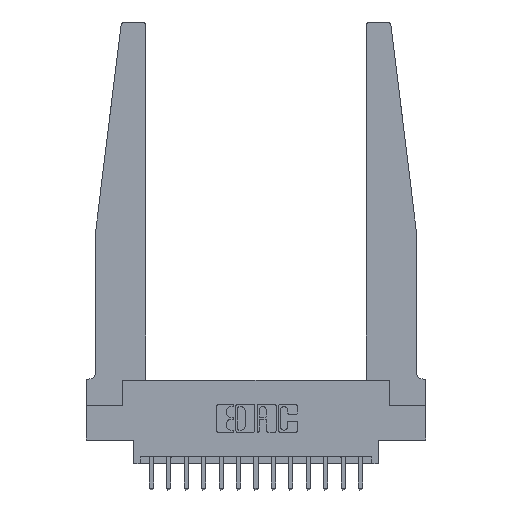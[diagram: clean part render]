
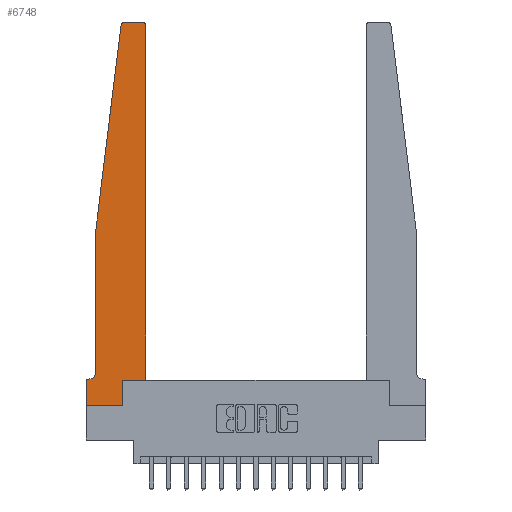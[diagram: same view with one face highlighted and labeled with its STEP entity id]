
A CAD part, top view. The second image highlights one B-rep face of the part: STEP entity #6748.
In plain terms, the highlighted planar face has unit normal (0, 0, 1).
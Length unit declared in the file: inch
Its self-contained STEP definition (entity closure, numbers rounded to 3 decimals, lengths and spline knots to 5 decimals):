
#84 = VERTEX_POINT ( 'NONE', #8165 ) ;
#368 = ORIENTED_EDGE ( 'NONE', *, *, #16164, .T. ) ;
#447 = VERTEX_POINT ( 'NONE', #3151 ) ;
#698 = CARTESIAN_POINT ( 'NONE',  ( 0.065, 0.1875, 0.37 ) ) ;
#712 = CARTESIAN_POINT ( 'NONE',  ( 0.27653, 2.75, 0.37 ) ) ;
#878 = EDGE_CURVE ( 'NONE', #8238, #4506, #9283, .T. ) ;
#1342 = DIRECTION ( 'NONE',  ( 1., 0., 0. ) ) ;
#1402 = AXIS2_PLACEMENT_3D ( 'NONE', #2797, #12107, #4126 ) ;
#1645 = ORIENTED_EDGE ( 'NONE', *, *, #16188, .T. ) ;
#1782 = CARTESIAN_POINT ( 'NONE',  ( 0.25, 2.75, 0.37 ) ) ;
#2006 = EDGE_CURVE ( 'NONE', #3058, #6667, #7144, .T. ) ;
#2750 = CARTESIAN_POINT ( 'NONE',  ( 0.425, 0.18, 0.37 ) ) ;
#2772 = CARTESIAN_POINT ( 'NONE',  ( 0., 0., 0.37 ) ) ;
#2797 = CARTESIAN_POINT ( 'NONE',  ( 0., 0.1875, 0.37 ) ) ;
#3058 = VERTEX_POINT ( 'NONE', #8673 ) ;
#3151 = CARTESIAN_POINT ( 'NONE',  ( 0.015, 0.1875, 0.37 ) ) ;
#3256 = DIRECTION ( 'NONE',  ( 1., 0., 0. ) ) ;
#4053 = EDGE_CURVE ( 'NONE', #12552, #5627, #13648, .T. ) ;
#4085 = DIRECTION ( 'NONE',  ( 0., 1., 0. ) ) ;
#4126 = DIRECTION ( 'NONE',  ( 1., 0., 0. ) ) ;
#4337 = ORIENTED_EDGE ( 'NONE', *, *, #11770, .T. ) ;
#4506 = VERTEX_POINT ( 'NONE', #17321 ) ;
#4568 = AXIS2_PLACEMENT_3D ( 'NONE', #10434, #10341, #10271 ) ;
#4741 = CIRCLE ( 'NONE', #15214, 0.05 ) ;
#4788 = EDGE_LOOP ( 'NONE', ( #9194, #16767, #4337, #1645, #368, #7497, #8402, #14737, #12837, #5644, #10534, #6061 ) ) ;
#4977 = DIRECTION ( 'NONE',  ( 0., 0., -1. ) ) ;
#5025 = CARTESIAN_POINT ( 'NONE',  ( 0., 0.1875, 0.37 ) ) ;
#5384 = CARTESIAN_POINT ( 'NONE',  ( 0.065, 1.25, 0.37 ) ) ;
#5473 = VERTEX_POINT ( 'NONE', #5384 ) ;
#5627 = VERTEX_POINT ( 'NONE', #12434 ) ;
#5644 = ORIENTED_EDGE ( 'NONE', *, *, #14014, .T. ) ;
#6061 = ORIENTED_EDGE ( 'NONE', *, *, #2006, .T. ) ;
#6319 = CARTESIAN_POINT ( 'NONE',  ( 0.425, 0.18, 0.37 ) ) ;
#6344 = CARTESIAN_POINT ( 'NONE',  ( 0.065, 1.25, 0.37 ) ) ;
#6378 = CARTESIAN_POINT ( 'NONE',  ( 0.27653, 2.72, 0.37 ) ) ;
#6637 = CARTESIAN_POINT ( 'NONE',  ( 0.2605, 0.18, 0.37 ) ) ;
#6667 = VERTEX_POINT ( 'NONE', #17427 ) ;
#6748 = ADVANCED_FACE ( 'NONE', ( #12920 ), #10867, .T. ) ;
#6794 = LINE ( 'NONE', #11436, #9954 ) ;
#7144 = CIRCLE ( 'NONE', #4568, 0.03 ) ;
#7202 = VECTOR ( 'NONE', #9821, 39.37008 ) ;
#7497 = ORIENTED_EDGE ( 'NONE', *, *, #16722, .T. ) ;
#7682 = DIRECTION ( 'NONE',  ( 0., -1., 0. ) ) ;
#7914 = VECTOR ( 'NONE', #7682, 39.37008 ) ;
#8006 = EDGE_CURVE ( 'NONE', #5627, #84, #16584, .T. ) ;
#8161 = DIRECTION ( 'NONE',  ( 0., -1., 0. ) ) ;
#8165 = CARTESIAN_POINT ( 'NONE',  ( 0.2605, 0., 0.37 ) ) ;
#8238 = VERTEX_POINT ( 'NONE', #712 ) ;
#8402 = ORIENTED_EDGE ( 'NONE', *, *, #4053, .T. ) ;
#8673 = CARTESIAN_POINT ( 'NONE',  ( 0.425, 2.72, 0.37 ) ) ;
#8734 = LINE ( 'NONE', #2750, #15506 ) ;
#8839 = CARTESIAN_POINT ( 'NONE',  ( 0.2605, 0.18, 0.37 ) ) ;
#9194 = ORIENTED_EDGE ( 'NONE', *, *, #12276, .T. ) ;
#9283 = CIRCLE ( 'NONE', #14992, 0.03 ) ;
#9821 = DIRECTION ( 'NONE',  ( -1., 0., 0. ) ) ;
#9954 = VECTOR ( 'NONE', #15510, 39.37008 ) ;
#10111 = DIRECTION ( 'NONE',  ( 0., 0., 1. ) ) ;
#10227 = LINE ( 'NONE', #698, #16954 ) ;
#10271 = DIRECTION ( 'NONE',  ( 1., 0., 0. ) ) ;
#10341 = DIRECTION ( 'NONE',  ( 0., 0., 1. ) ) ;
#10417 = EDGE_CURVE ( 'NONE', #15129, #3058, #8734, .T. ) ;
#10434 = CARTESIAN_POINT ( 'NONE',  ( 0.395, 2.72, 0.37 ) ) ;
#10534 = ORIENTED_EDGE ( 'NONE', *, *, #10417, .T. ) ;
#10815 = LINE ( 'NONE', #1782, #7202 ) ;
#10867 = PLANE ( 'NONE',  #1402 ) ;
#11160 = CARTESIAN_POINT ( 'NONE',  ( 0., 0., 0.37 ) ) ;
#11436 = CARTESIAN_POINT ( 'NONE',  ( 0.065, 1.25, 0.37 ) ) ;
#11512 = LINE ( 'NONE', #6344, #7914 ) ;
#11770 = EDGE_CURVE ( 'NONE', #4506, #5473, #6794, .T. ) ;
#12030 = EDGE_CURVE ( 'NONE', #84, #16758, #14175, .T. ) ;
#12107 = DIRECTION ( 'NONE',  ( 0., 0., 1. ) ) ;
#12276 = EDGE_CURVE ( 'NONE', #6667, #8238, #10815, .T. ) ;
#12434 = CARTESIAN_POINT ( 'NONE',  ( 0., 0., 0.37 ) ) ;
#12552 = VERTEX_POINT ( 'NONE', #5025 ) ;
#12837 = ORIENTED_EDGE ( 'NONE', *, *, #12030, .T. ) ;
#12920 = FACE_OUTER_BOUND ( 'NONE', #4788, .T. ) ;
#13018 = VECTOR ( 'NONE', #16559, 39.37008 ) ;
#13070 = CARTESIAN_POINT ( 'NONE',  ( 0.015, 0.2375, 0.37 ) ) ;
#13214 = VECTOR ( 'NONE', #8161, 39.37008 ) ;
#13380 = CARTESIAN_POINT ( 'NONE',  ( 0.425, 0.18, 0.37 ) ) ;
#13648 = LINE ( 'NONE', #2772, #13214 ) ;
#13696 = VECTOR ( 'NONE', #1342, 39.37008 ) ;
#13759 = VECTOR ( 'NONE', #17411, 39.37008 ) ;
#14014 = EDGE_CURVE ( 'NONE', #16758, #15129, #17251, .T. ) ;
#14175 = LINE ( 'NONE', #6637, #13759 ) ;
#14433 = DIRECTION ( 'NONE',  ( -1., 0., 0. ) ) ;
#14737 = ORIENTED_EDGE ( 'NONE', *, *, #8006, .T. ) ;
#14992 = AXIS2_PLACEMENT_3D ( 'NONE', #6378, #10111, #3256 ) ;
#15129 = VERTEX_POINT ( 'NONE', #6319 ) ;
#15181 = CARTESIAN_POINT ( 'NONE',  ( 0.065, 0.2375, 0.37 ) ) ;
#15214 = AXIS2_PLACEMENT_3D ( 'NONE', #13070, #4977, #14433 ) ;
#15463 = VERTEX_POINT ( 'NONE', #15181 ) ;
#15506 = VECTOR ( 'NONE', #4085, 39.37008 ) ;
#15510 = DIRECTION ( 'NONE',  ( -0.122, -0.992, 0. ) ) ;
#16164 = EDGE_CURVE ( 'NONE', #15463, #447, #4741, .T. ) ;
#16188 = EDGE_CURVE ( 'NONE', #5473, #15463, #11512, .T. ) ;
#16559 = DIRECTION ( 'NONE',  ( 1., 0., 0. ) ) ;
#16584 = LINE ( 'NONE', #11160, #13018 ) ;
#16722 = EDGE_CURVE ( 'NONE', #447, #12552, #10227, .T. ) ;
#16758 = VERTEX_POINT ( 'NONE', #8839 ) ;
#16767 = ORIENTED_EDGE ( 'NONE', *, *, #878, .T. ) ;
#16777 = DIRECTION ( 'NONE',  ( -1., 0., 0. ) ) ;
#16954 = VECTOR ( 'NONE', #16777, 39.37008 ) ;
#17251 = LINE ( 'NONE', #13380, #13696 ) ;
#17321 = CARTESIAN_POINT ( 'NONE',  ( 0.24675, 2.72367, 0.37 ) ) ;
#17411 = DIRECTION ( 'NONE',  ( 0., 1., 0. ) ) ;
#17427 = CARTESIAN_POINT ( 'NONE',  ( 0.395, 2.75, 0.37 ) ) ;
